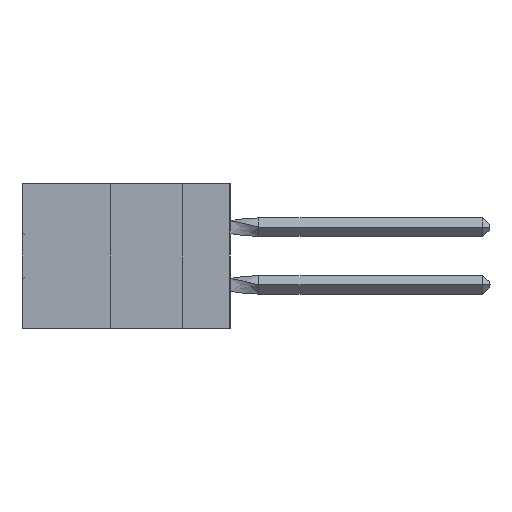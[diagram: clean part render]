
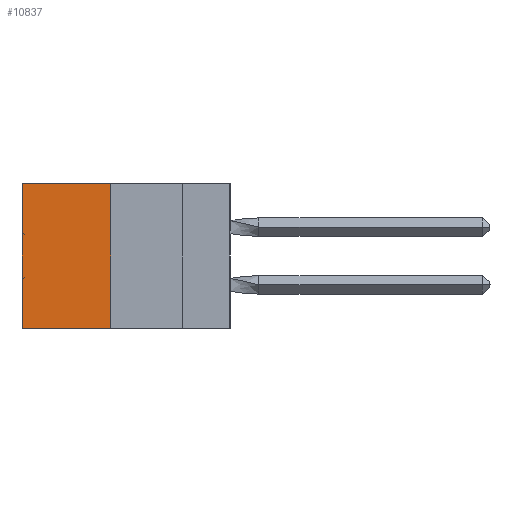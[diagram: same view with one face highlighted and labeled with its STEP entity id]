
A CAD part, left-side view. The second image highlights one B-rep face of the part: STEP entity #10837.
In plain terms, the highlighted planar face has unit normal (-1, 0, 0).
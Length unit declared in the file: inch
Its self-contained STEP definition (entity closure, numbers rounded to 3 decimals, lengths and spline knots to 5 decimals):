
#32 = VERTEX_POINT ( 'NONE', #9804 ) ;
#2150 = CARTESIAN_POINT ( 'NONE',  ( 0.305, 0.413, -0.5 ) ) ;
#4808 = FACE_OUTER_BOUND ( 'NONE', #23013, .T. ) ;
#5835 = VECTOR ( 'NONE', #51521, 39.37008 ) ;
#6038 = EDGE_CURVE ( 'NONE', #29202, #44085, #46299, .T. ) ;
#7160 = EDGE_CURVE ( 'NONE', #29202, #44998, #52844, .T. ) ;
#8398 = ORIENTED_EDGE ( 'NONE', *, *, #6038, .F. ) ;
#9804 = CARTESIAN_POINT ( 'NONE',  ( 0.305, 0.72, -0.5 ) ) ;
#10837 = ADVANCED_FACE ( 'NONE', ( #4808 ), #19144, .F. ) ;
#11152 = DIRECTION ( 'NONE',  ( 0., 1., 0. ) ) ;
#14430 = CARTESIAN_POINT ( 'NONE',  ( 0.305, 0.72, 0. ) ) ;
#15140 = DIRECTION ( 'NONE',  ( 0., 1., 0. ) ) ;
#19144 = PLANE ( 'NONE',  #25780 ) ;
#21088 = LINE ( 'NONE', #2150, #53739 ) ;
#22214 = VECTOR ( 'NONE', #34819, 39.37008 ) ;
#22640 = ORIENTED_EDGE ( 'NONE', *, *, #47579, .F. ) ;
#23013 = EDGE_LOOP ( 'NONE', ( #26568, #22640, #8398, #31016 ) ) ;
#25780 = AXIS2_PLACEMENT_3D ( 'NONE', #48932, #45962, #29689 ) ;
#26568 = ORIENTED_EDGE ( 'NONE', *, *, #27104, .T. ) ;
#27104 = EDGE_CURVE ( 'NONE', #44998, #32, #33891, .T. ) ;
#29202 = VERTEX_POINT ( 'NONE', #34623 ) ;
#29225 = CARTESIAN_POINT ( 'NONE',  ( 0.305, 0.413, -0.5 ) ) ;
#29689 = DIRECTION ( 'NONE',  ( 0., 0., -1. ) ) ;
#30488 = CARTESIAN_POINT ( 'NONE',  ( 0.305, 0.72, -0.5 ) ) ;
#31016 = ORIENTED_EDGE ( 'NONE', *, *, #7160, .T. ) ;
#33891 = LINE ( 'NONE', #30488, #5835 ) ;
#34623 = CARTESIAN_POINT ( 'NONE',  ( 0.305, 0.413, 0. ) ) ;
#34685 = CARTESIAN_POINT ( 'NONE',  ( 0.305, 0.413, 0. ) ) ;
#34819 = DIRECTION ( 'NONE',  ( 0., 0., -1. ) ) ;
#39034 = CARTESIAN_POINT ( 'NONE',  ( 0.305, 0.413, -0.5 ) ) ;
#41742 = VECTOR ( 'NONE', #11152, 39.37008 ) ;
#44085 = VERTEX_POINT ( 'NONE', #29225 ) ;
#44998 = VERTEX_POINT ( 'NONE', #14430 ) ;
#45962 = DIRECTION ( 'NONE',  ( 1., 0., 0. ) ) ;
#46299 = LINE ( 'NONE', #39034, #22214 ) ;
#47579 = EDGE_CURVE ( 'NONE', #44085, #32, #21088, .T. ) ;
#48932 = CARTESIAN_POINT ( 'NONE',  ( 0.305, 0.413, -0.5 ) ) ;
#51521 = DIRECTION ( 'NONE',  ( 0., 0., -1. ) ) ;
#52844 = LINE ( 'NONE', #34685, #41742 ) ;
#53739 = VECTOR ( 'NONE', #15140, 39.37008 ) ;
